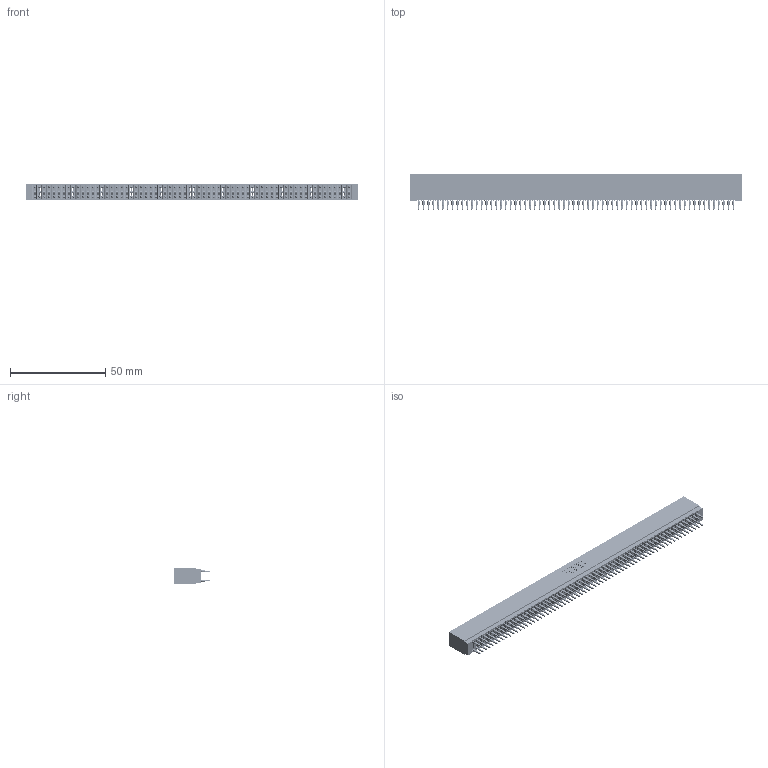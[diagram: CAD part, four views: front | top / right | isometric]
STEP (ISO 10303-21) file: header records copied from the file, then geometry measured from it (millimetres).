
FILE_DESCRIPTION (( 'STEP AP203' ), '1' );
FILE_NAME ('725-132-560-201.STEP', '2020-09-10T11:23:24', ( '' ), ( '' ), 'SwSTEP 2.0', 'SolidWorks 2020', '' );
FILE_SCHEMA (( 'CONFIG_CONTROL_DESIGN' ));
Length unit declared in the file: inch
Products named in the file (3): 745-292-001_560; 725 Part_Insulator Option - 01; 725-132-560-201
Assembly tree (133 placements, depth 2):
  725-132-560-201
    725 Part_Insulator Option - 01
    745-292-001_560  x132
Bounding box: 174.24 x 18.81 x 8.89 mm (x, y, z)
Volume: 14185.1 mm3; surface area: 32558.2 mm2
Topology: 133 solids, 133 shells, 13097 faces, 35828 edges, 22740 vertices
Faces by surface type: plane 6787, cylinder 2878, bspline 2640, torus 792
Entity records: 108129 total; most frequent: CARTESIAN_POINT 19249, ORIENTED_EDGE 18732, DIRECTION 16350, EDGE_CURVE 9366, VECTOR 8780, LINE 8780, VERTEX_POINT 5972, AXIS2_PLACEMENT_3D 3785
